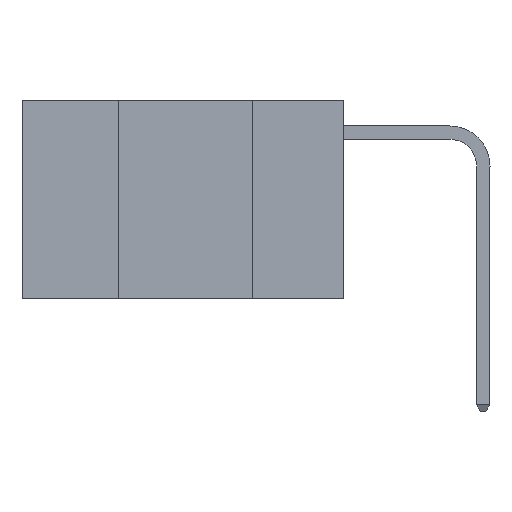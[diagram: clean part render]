
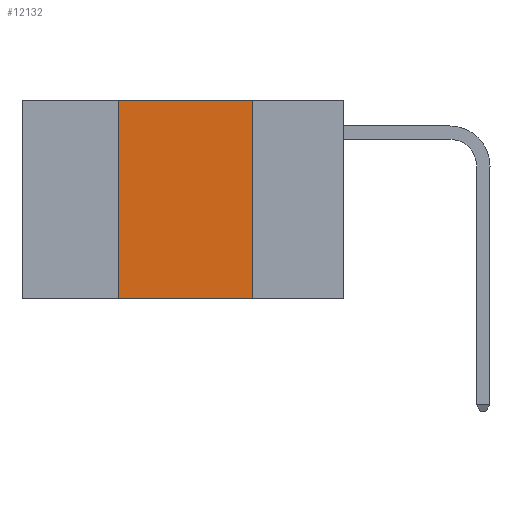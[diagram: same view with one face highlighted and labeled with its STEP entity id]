
A CAD part, left-side view. The second image highlights one B-rep face of the part: STEP entity #12132.
In plain terms, the highlighted planar face has unit normal (-1, 0, 0).
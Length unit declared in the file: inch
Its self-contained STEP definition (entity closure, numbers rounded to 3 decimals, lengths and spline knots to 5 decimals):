
#197 = DIRECTION ( 'NONE',  ( 0., 0., -1. ) ) ;
#375 = VERTEX_POINT ( 'NONE', #1673 ) ;
#1184 = DIRECTION ( 'NONE',  ( 0., 0., -1. ) ) ;
#1673 = CARTESIAN_POINT ( 'NONE',  ( 0., 0.42, -0.37 ) ) ;
#2331 = FACE_OUTER_BOUND ( 'NONE', #6337, .T. ) ;
#2448 = VECTOR ( 'NONE', #14150, 39.37008 ) ;
#4545 = CARTESIAN_POINT ( 'NONE',  ( 0., 0.6, -0.37 ) ) ;
#5162 = DIRECTION ( 'NONE',  ( 0., -1., 0. ) ) ;
#5322 = EDGE_CURVE ( 'NONE', #375, #10046, #16200, .T. ) ;
#5698 = LINE ( 'NONE', #6029, #2448 ) ;
#5801 = LINE ( 'NONE', #8095, #13032 ) ;
#6029 = CARTESIAN_POINT ( 'NONE',  ( 0., 0.42, 0. ) ) ;
#6337 = EDGE_LOOP ( 'NONE', ( #14989, #9265, #7952, #17721 ) ) ;
#7123 = PLANE ( 'NONE',  #9112 ) ;
#7361 = EDGE_CURVE ( 'NONE', #10484, #8164, #14234, .T. ) ;
#7610 = CARTESIAN_POINT ( 'NONE',  ( 0., 0.17, -0.37 ) ) ;
#7952 = ORIENTED_EDGE ( 'NONE', *, *, #8304, .F. ) ;
#8095 = CARTESIAN_POINT ( 'NONE',  ( 0., 0.17, 0. ) ) ;
#8164 = VERTEX_POINT ( 'NONE', #14965 ) ;
#8304 = EDGE_CURVE ( 'NONE', #375, #10484, #5698, .T. ) ;
#8516 = DIRECTION ( 'NONE',  ( 1., 0., 0. ) ) ;
#9112 = AXIS2_PLACEMENT_3D ( 'NONE', #9805, #8516, #197 ) ;
#9265 = ORIENTED_EDGE ( 'NONE', *, *, #7361, .F. ) ;
#9805 = CARTESIAN_POINT ( 'NONE',  ( 0., 0.6, 0. ) ) ;
#10046 = VERTEX_POINT ( 'NONE', #7610 ) ;
#10484 = VERTEX_POINT ( 'NONE', #14177 ) ;
#10586 = CARTESIAN_POINT ( 'NONE',  ( 0., 0.6, 0. ) ) ;
#11959 = EDGE_CURVE ( 'NONE', #8164, #10046, #5801, .T. ) ;
#12132 = ADVANCED_FACE ( 'NONE', ( #2331 ), #7123, .F. ) ;
#13032 = VECTOR ( 'NONE', #1184, 39.37008 ) ;
#13794 = VECTOR ( 'NONE', #5162, 39.37008 ) ;
#14150 = DIRECTION ( 'NONE',  ( 0., 0., 1. ) ) ;
#14177 = CARTESIAN_POINT ( 'NONE',  ( 0., 0.42, 0. ) ) ;
#14234 = LINE ( 'NONE', #10586, #13794 ) ;
#14965 = CARTESIAN_POINT ( 'NONE',  ( 0., 0.17, 0. ) ) ;
#14989 = ORIENTED_EDGE ( 'NONE', *, *, #11959, .F. ) ;
#15789 = VECTOR ( 'NONE', #16759, 39.37008 ) ;
#16200 = LINE ( 'NONE', #4545, #15789 ) ;
#16759 = DIRECTION ( 'NONE',  ( 0., -1., 0. ) ) ;
#17721 = ORIENTED_EDGE ( 'NONE', *, *, #5322, .T. ) ;
